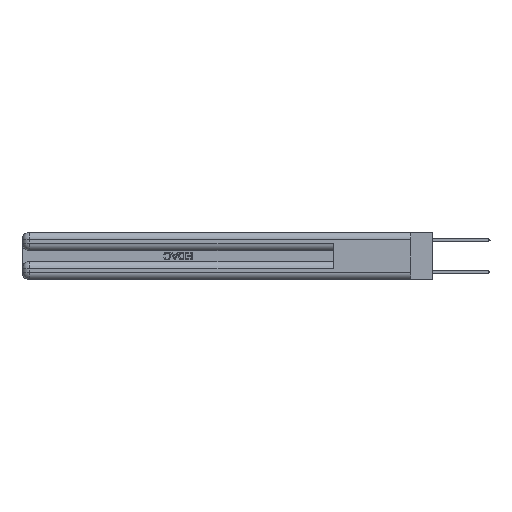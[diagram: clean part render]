
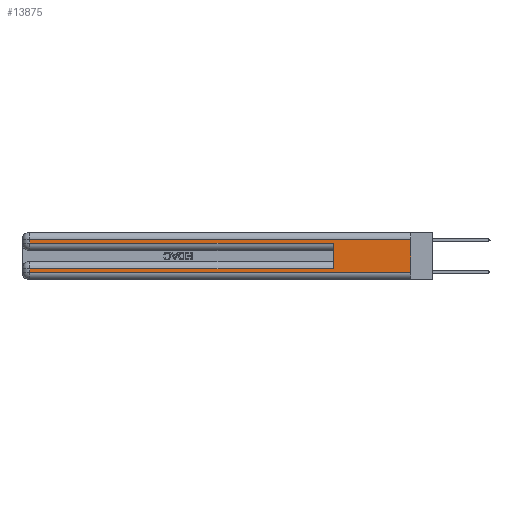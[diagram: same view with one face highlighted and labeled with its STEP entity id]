
A CAD part, left-side view. The second image highlights one B-rep face of the part: STEP entity #13875.
In plain terms, the highlighted planar face has unit normal (-1, 0, 0).
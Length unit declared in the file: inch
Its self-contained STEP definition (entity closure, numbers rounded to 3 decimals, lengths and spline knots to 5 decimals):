
#62 = VECTOR ( 'NONE', #9511, 39.37008 ) ;
#739 = ORIENTED_EDGE ( 'NONE', *, *, #30047, .T. ) ;
#909 = VERTEX_POINT ( 'NONE', #31852 ) ;
#2304 = CARTESIAN_POINT ( 'NONE',  ( 0., 2.94, 0.085 ) ) ;
#3395 = CARTESIAN_POINT ( 'NONE',  ( 0., 2.94, 0.37 ) ) ;
#3404 = EDGE_CURVE ( 'NONE', #10893, #10759, #23253, .T. ) ;
#3860 = DIRECTION ( 'NONE',  ( 0., 0., -1. ) ) ;
#4885 = CARTESIAN_POINT ( 'NONE',  ( 0., 0.6, 0.145 ) ) ;
#4962 = EDGE_LOOP ( 'NONE', ( #29905, #27634, #739, #13565, #32128, #29625, #33242, #19759 ) ) ;
#5051 = CARTESIAN_POINT ( 'NONE',  ( 0., 0., 0.285 ) ) ;
#5288 = EDGE_CURVE ( 'NONE', #27666, #10759, #13933, .T. ) ;
#6724 = CARTESIAN_POINT ( 'NONE',  ( 0., 0., 0.31 ) ) ;
#6899 = CARTESIAN_POINT ( 'NONE',  ( 0., 2.94, 0.285 ) ) ;
#7221 = LINE ( 'NONE', #3395, #20235 ) ;
#7707 = DIRECTION ( 'NONE',  ( 0., 0., 1. ) ) ;
#7756 = DIRECTION ( 'NONE',  ( 1., 0., 0. ) ) ;
#8540 = VECTOR ( 'NONE', #7707, 39.37008 ) ;
#9032 = EDGE_CURVE ( 'NONE', #10893, #27925, #25773, .T. ) ;
#9360 = CARTESIAN_POINT ( 'NONE',  ( 0., 2.94, 0.37 ) ) ;
#9511 = DIRECTION ( 'NONE',  ( 0., 1., 0. ) ) ;
#10759 = VERTEX_POINT ( 'NONE', #27476 ) ;
#10893 = VERTEX_POINT ( 'NONE', #28435 ) ;
#11986 = VECTOR ( 'NONE', #15876, 39.37008 ) ;
#12769 = EDGE_CURVE ( 'NONE', #27925, #27748, #7221, .T. ) ;
#13565 = ORIENTED_EDGE ( 'NONE', *, *, #5288, .T. ) ;
#13875 = ADVANCED_FACE ( 'NONE', ( #30432 ), #18802, .F. ) ;
#13933 = LINE ( 'NONE', #5051, #34990 ) ;
#14346 = LINE ( 'NONE', #26613, #19966 ) ;
#14482 = DIRECTION ( 'NONE',  ( 0., 0., -1. ) ) ;
#14590 = VERTEX_POINT ( 'NONE', #21901 ) ;
#14803 = VECTOR ( 'NONE', #3860, 39.37008 ) ;
#14961 = LINE ( 'NONE', #6724, #62 ) ;
#15647 = CARTESIAN_POINT ( 'NONE',  ( 0., 2.94, 0.06 ) ) ;
#15876 = DIRECTION ( 'NONE',  ( 0., 1., 0. ) ) ;
#18225 = VECTOR ( 'NONE', #32744, 39.37008 ) ;
#18344 = EDGE_CURVE ( 'NONE', #27748, #909, #32799, .T. ) ;
#18802 = PLANE ( 'NONE',  #29275 ) ;
#19759 = ORIENTED_EDGE ( 'NONE', *, *, #18344, .T. ) ;
#19966 = VECTOR ( 'NONE', #32111, 39.37008 ) ;
#20235 = VECTOR ( 'NONE', #14482, 39.37008 ) ;
#21811 = DIRECTION ( 'NONE',  ( 0., -1., 0. ) ) ;
#21901 = CARTESIAN_POINT ( 'NONE',  ( 0., 2.94, 0.31 ) ) ;
#22184 = LINE ( 'NONE', #9360, #14803 ) ;
#23253 = LINE ( 'NONE', #4885, #8540 ) ;
#24323 = CARTESIAN_POINT ( 'NONE',  ( 0., 0., 0.37 ) ) ;
#24552 = EDGE_CURVE ( 'NONE', #35651, #909, #14346, .T. ) ;
#25577 = CARTESIAN_POINT ( 'NONE',  ( 0., 0., 0.31 ) ) ;
#25773 = LINE ( 'NONE', #32317, #11986 ) ;
#26613 = CARTESIAN_POINT ( 'NONE',  ( 0., 0., 0.37 ) ) ;
#27072 = DIRECTION ( 'NONE',  ( 0., 0., -1. ) ) ;
#27243 = CARTESIAN_POINT ( 'NONE',  ( 0., 0., 0.06 ) ) ;
#27476 = CARTESIAN_POINT ( 'NONE',  ( 0., 0.6, 0.285 ) ) ;
#27634 = ORIENTED_EDGE ( 'NONE', *, *, #33718, .T. ) ;
#27666 = VERTEX_POINT ( 'NONE', #6899 ) ;
#27748 = VERTEX_POINT ( 'NONE', #15647 ) ;
#27925 = VERTEX_POINT ( 'NONE', #2304 ) ;
#28435 = CARTESIAN_POINT ( 'NONE',  ( 0., 0.6, 0.085 ) ) ;
#29275 = AXIS2_PLACEMENT_3D ( 'NONE', #24323, #7756, #27072 ) ;
#29625 = ORIENTED_EDGE ( 'NONE', *, *, #9032, .T. ) ;
#29905 = ORIENTED_EDGE ( 'NONE', *, *, #24552, .F. ) ;
#30047 = EDGE_CURVE ( 'NONE', #14590, #27666, #22184, .T. ) ;
#30432 = FACE_OUTER_BOUND ( 'NONE', #4962, .T. ) ;
#31852 = CARTESIAN_POINT ( 'NONE',  ( 0., 0., 0.06 ) ) ;
#32111 = DIRECTION ( 'NONE',  ( 0., 0., -1. ) ) ;
#32128 = ORIENTED_EDGE ( 'NONE', *, *, #3404, .F. ) ;
#32317 = CARTESIAN_POINT ( 'NONE',  ( 0., 0., 0.085 ) ) ;
#32744 = DIRECTION ( 'NONE',  ( 0., -1., 0. ) ) ;
#32799 = LINE ( 'NONE', #27243, #18225 ) ;
#33242 = ORIENTED_EDGE ( 'NONE', *, *, #12769, .T. ) ;
#33718 = EDGE_CURVE ( 'NONE', #35651, #14590, #14961, .T. ) ;
#34990 = VECTOR ( 'NONE', #21811, 39.37008 ) ;
#35651 = VERTEX_POINT ( 'NONE', #25577 ) ;
